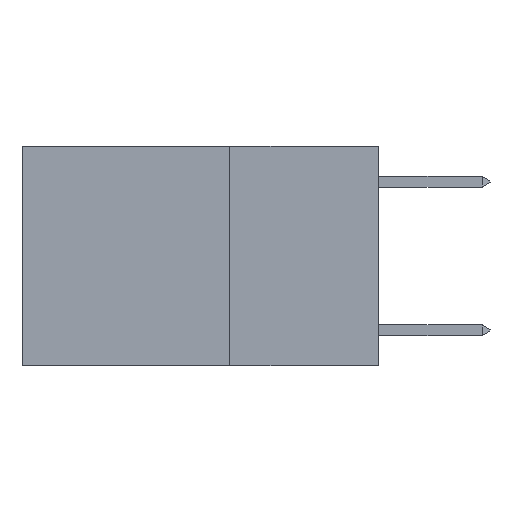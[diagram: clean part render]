
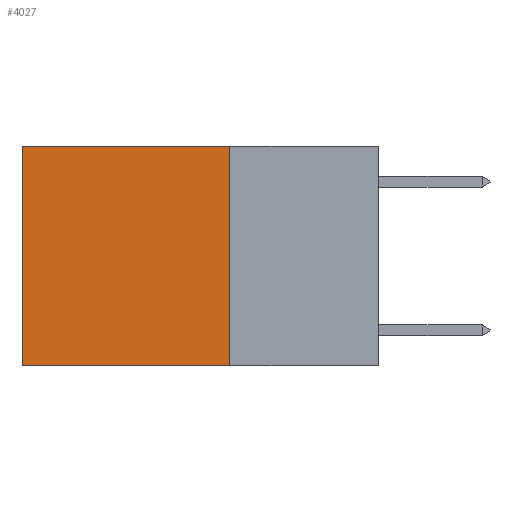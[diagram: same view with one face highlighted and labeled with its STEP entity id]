
A CAD part, left-side view. The second image highlights one B-rep face of the part: STEP entity #4027.
In plain terms, the highlighted planar face has unit normal (-1, 0, 0).
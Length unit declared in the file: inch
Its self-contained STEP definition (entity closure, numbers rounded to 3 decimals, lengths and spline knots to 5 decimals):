
#214 = DIRECTION ( 'NONE',  ( 1., 0., 0. ) ) ;
#287 = AXIS2_PLACEMENT_3D ( 'NONE', #7697, #214, #3128 ) ;
#384 = VERTEX_POINT ( 'NONE', #7629 ) ;
#527 = CARTESIAN_POINT ( 'NONE',  ( 0.2625, 0.25, -0.37 ) ) ;
#528 = CARTESIAN_POINT ( 'NONE',  ( 0.2625, 0.25, 0. ) ) ;
#762 = EDGE_CURVE ( 'NONE', #10340, #384, #8795, .T. ) ;
#844 = EDGE_CURVE ( 'NONE', #7059, #10340, #5234, .T. ) ;
#939 = EDGE_LOOP ( 'NONE', ( #3282, #5707, #2243, #7955 ) ) ;
#1178 = VECTOR ( 'NONE', #7991, 39.37008 ) ;
#1386 = VECTOR ( 'NONE', #2467, 39.37008 ) ;
#1429 = CARTESIAN_POINT ( 'NONE',  ( 0.2625, 0.25, 0. ) ) ;
#1995 = LINE ( 'NONE', #528, #2913 ) ;
#2192 = CARTESIAN_POINT ( 'NONE',  ( 0.2625, 0.25, 0. ) ) ;
#2243 = ORIENTED_EDGE ( 'NONE', *, *, #844, .F. ) ;
#2467 = DIRECTION ( 'NONE',  ( 0., 1., 0. ) ) ;
#2870 = LINE ( 'NONE', #3962, #3941 ) ;
#2913 = VECTOR ( 'NONE', #6140, 39.37008 ) ;
#3128 = DIRECTION ( 'NONE',  ( 0., 0., -1. ) ) ;
#3231 = EDGE_CURVE ( 'NONE', #3332, #384, #2870, .T. ) ;
#3282 = ORIENTED_EDGE ( 'NONE', *, *, #3231, .T. ) ;
#3332 = VERTEX_POINT ( 'NONE', #9817 ) ;
#3941 = VECTOR ( 'NONE', #7504, 39.37008 ) ;
#3962 = CARTESIAN_POINT ( 'NONE',  ( 0.2625, 0.6, 0. ) ) ;
#4027 = ADVANCED_FACE ( 'NONE', ( #7356 ), #7529, .F. ) ;
#4352 = EDGE_CURVE ( 'NONE', #7059, #3332, #1995, .T. ) ;
#5234 = LINE ( 'NONE', #1429, #1178 ) ;
#5707 = ORIENTED_EDGE ( 'NONE', *, *, #762, .F. ) ;
#6140 = DIRECTION ( 'NONE',  ( 0., 1., 0. ) ) ;
#7059 = VERTEX_POINT ( 'NONE', #2192 ) ;
#7356 = FACE_OUTER_BOUND ( 'NONE', #939, .T. ) ;
#7504 = DIRECTION ( 'NONE',  ( 0., 0., -1. ) ) ;
#7529 = PLANE ( 'NONE',  #287 ) ;
#7629 = CARTESIAN_POINT ( 'NONE',  ( 0.2625, 0.6, -0.37 ) ) ;
#7697 = CARTESIAN_POINT ( 'NONE',  ( 0.2625, 0.25, 0. ) ) ;
#7955 = ORIENTED_EDGE ( 'NONE', *, *, #4352, .T. ) ;
#7991 = DIRECTION ( 'NONE',  ( 0., 0., -1. ) ) ;
#8795 = LINE ( 'NONE', #527, #1386 ) ;
#9817 = CARTESIAN_POINT ( 'NONE',  ( 0.2625, 0.6, 0. ) ) ;
#10340 = VERTEX_POINT ( 'NONE', #10448 ) ;
#10448 = CARTESIAN_POINT ( 'NONE',  ( 0.2625, 0.25, -0.37 ) ) ;
